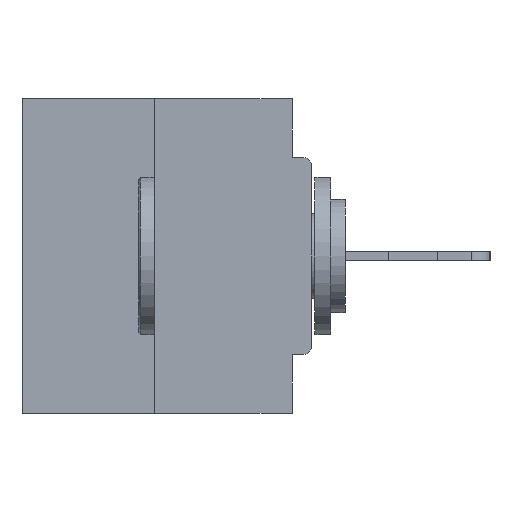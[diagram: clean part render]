
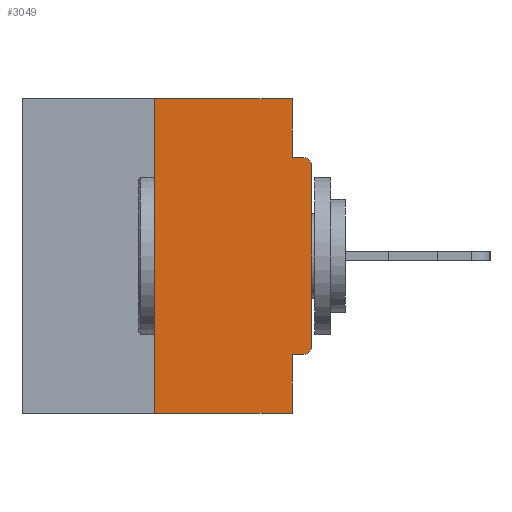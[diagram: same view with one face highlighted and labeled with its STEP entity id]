
A CAD part, left-side view. The second image highlights one B-rep face of the part: STEP entity #3049.
In plain terms, the highlighted planar face has unit normal (-1, 0, 0).
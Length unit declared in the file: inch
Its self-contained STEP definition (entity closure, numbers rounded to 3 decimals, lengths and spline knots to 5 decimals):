
#27 = DIRECTION ( 'NONE',  ( -1., 0., 0. ) ) ;
#231 = ORIENTED_EDGE ( 'NONE', *, *, #7795, .F. ) ;
#780 = VERTEX_POINT ( 'NONE', #21544 ) ;
#1097 = CARTESIAN_POINT ( 'NONE',  ( 0., 0., -0.1085 ) ) ;
#1395 = DIRECTION ( 'NONE',  ( 0., 1., 0. ) ) ;
#1961 = VERTEX_POINT ( 'NONE', #17027 ) ;
#2012 = ORIENTED_EDGE ( 'NONE', *, *, #29694, .F. ) ;
#2595 = AXIS2_PLACEMENT_3D ( 'NONE', #8878, #22515, #6292 ) ;
#3049 = ADVANCED_FACE ( 'NONE', ( #29610 ), #13852, .F. ) ;
#3472 = CIRCLE ( 'NONE', #5895, 0.015 ) ;
#3788 = CARTESIAN_POINT ( 'NONE',  ( 0., 0., -0.0935 ) ) ;
#3988 = VECTOR ( 'NONE', #19662, 39.37008 ) ;
#4588 = CARTESIAN_POINT ( 'NONE',  ( 0., 0.015, -0.1085 ) ) ;
#4682 = CARTESIAN_POINT ( 'NONE',  ( 0., 0.25, 0. ) ) ;
#4723 = DIRECTION ( 'NONE',  ( 0., 0., -1. ) ) ;
#5309 = VECTOR ( 'NONE', #21109, 39.37008 ) ;
#5895 = AXIS2_PLACEMENT_3D ( 'NONE', #4588, #27, #4723 ) ;
#6025 = LINE ( 'NONE', #24496, #24641 ) ;
#6292 = DIRECTION ( 'NONE',  ( 0., 0., -1. ) ) ;
#6522 = DIRECTION ( 'NONE',  ( 0., -1., 0. ) ) ;
#6960 = DIRECTION ( 'NONE',  ( 0., 0., 1. ) ) ;
#7469 = ORIENTED_EDGE ( 'NONE', *, *, #28873, .T. ) ;
#7495 = CARTESIAN_POINT ( 'NONE',  ( 0., 0.031, -0.5 ) ) ;
#7795 = EDGE_CURVE ( 'NONE', #17974, #28939, #20951, .T. ) ;
#8878 = CARTESIAN_POINT ( 'NONE',  ( 0., 0.015, -0.3915 ) ) ;
#8958 = VECTOR ( 'NONE', #6522, 39.37008 ) ;
#9535 = VERTEX_POINT ( 'NONE', #1097 ) ;
#9599 = CARTESIAN_POINT ( 'NONE',  ( 0., 0.46, 0. ) ) ;
#10550 = EDGE_CURVE ( 'NONE', #14853, #29250, #29198, .T. ) ;
#11734 = CARTESIAN_POINT ( 'NONE',  ( 0., 0.46, 0. ) ) ;
#12317 = ORIENTED_EDGE ( 'NONE', *, *, #26937, .T. ) ;
#13119 = DIRECTION ( 'NONE',  ( 0., 0., 1. ) ) ;
#13852 = PLANE ( 'NONE',  #20793 ) ;
#14151 = DIRECTION ( 'NONE',  ( 1., 0., 0. ) ) ;
#14847 = EDGE_CURVE ( 'NONE', #1961, #14853, #21865, .T. ) ;
#14853 = VERTEX_POINT ( 'NONE', #23837 ) ;
#15215 = LINE ( 'NONE', #26261, #18508 ) ;
#15325 = LINE ( 'NONE', #3788, #8958 ) ;
#15389 = EDGE_CURVE ( 'NONE', #17050, #28939, #6025, .T. ) ;
#15542 = LINE ( 'NONE', #15692, #16147 ) ;
#15692 = CARTESIAN_POINT ( 'NONE',  ( 0., 0., 0. ) ) ;
#15935 = CARTESIAN_POINT ( 'NONE',  ( 0., 0.25, -0.5 ) ) ;
#16147 = VECTOR ( 'NONE', #13119, 39.37008 ) ;
#16405 = VECTOR ( 'NONE', #16721, 39.37008 ) ;
#16721 = DIRECTION ( 'NONE',  ( 0., -1., 0. ) ) ;
#17027 = CARTESIAN_POINT ( 'NONE',  ( 0., 0.25, 0. ) ) ;
#17050 = VERTEX_POINT ( 'NONE', #15935 ) ;
#17974 = VERTEX_POINT ( 'NONE', #18708 ) ;
#17991 = DIRECTION ( 'NONE',  ( 0., -1., 0. ) ) ;
#18107 = CIRCLE ( 'NONE', #2595, 0.015 ) ;
#18137 = EDGE_CURVE ( 'NONE', #24770, #17974, #15215, .T. ) ;
#18480 = LINE ( 'NONE', #4682, #21465 ) ;
#18508 = VECTOR ( 'NONE', #1395, 39.37008 ) ;
#18692 = CARTESIAN_POINT ( 'NONE',  ( 0., 0.031, -0.5 ) ) ;
#18708 = CARTESIAN_POINT ( 'NONE',  ( 0., 0.031, -0.4065 ) ) ;
#18884 = EDGE_CURVE ( 'NONE', #17050, #1961, #18480, .T. ) ;
#19662 = DIRECTION ( 'NONE',  ( 0., 0., -1. ) ) ;
#20793 = AXIS2_PLACEMENT_3D ( 'NONE', #11734, #14151, #20970 ) ;
#20939 = VERTEX_POINT ( 'NONE', #27871 ) ;
#20951 = LINE ( 'NONE', #18692, #5309 ) ;
#20970 = DIRECTION ( 'NONE',  ( 0., 0., -1. ) ) ;
#21109 = DIRECTION ( 'NONE',  ( 0., 0., -1. ) ) ;
#21465 = VECTOR ( 'NONE', #6960, 39.37008 ) ;
#21544 = CARTESIAN_POINT ( 'NONE',  ( 0., 0., -0.3915 ) ) ;
#21865 = LINE ( 'NONE', #9599, #16405 ) ;
#22515 = DIRECTION ( 'NONE',  ( -1., 0., 0. ) ) ;
#23837 = CARTESIAN_POINT ( 'NONE',  ( 0., 0.031, 0. ) ) ;
#23899 = ORIENTED_EDGE ( 'NONE', *, *, #18884, .F. ) ;
#24052 = CARTESIAN_POINT ( 'NONE',  ( 0., 0.031, 0. ) ) ;
#24496 = CARTESIAN_POINT ( 'NONE',  ( 0., 0.46, -0.5 ) ) ;
#24641 = VECTOR ( 'NONE', #17991, 39.37008 ) ;
#24726 = CARTESIAN_POINT ( 'NONE',  ( 0., 0.031, -0.0935 ) ) ;
#24770 = VERTEX_POINT ( 'NONE', #27964 ) ;
#25485 = ORIENTED_EDGE ( 'NONE', *, *, #28832, .T. ) ;
#26261 = CARTESIAN_POINT ( 'NONE',  ( 0., 0., -0.4065 ) ) ;
#26679 = ORIENTED_EDGE ( 'NONE', *, *, #10550, .F. ) ;
#26937 = EDGE_CURVE ( 'NONE', #9535, #20939, #3472, .T. ) ;
#27421 = ORIENTED_EDGE ( 'NONE', *, *, #14847, .F. ) ;
#27871 = CARTESIAN_POINT ( 'NONE',  ( 0., 0.015, -0.0935 ) ) ;
#27964 = CARTESIAN_POINT ( 'NONE',  ( 0., 0.015, -0.4065 ) ) ;
#28832 = EDGE_CURVE ( 'NONE', #24770, #780, #18107, .T. ) ;
#28873 = EDGE_CURVE ( 'NONE', #780, #9535, #15542, .T. ) ;
#28939 = VERTEX_POINT ( 'NONE', #7495 ) ;
#28974 = ORIENTED_EDGE ( 'NONE', *, *, #18137, .F. ) ;
#29099 = EDGE_LOOP ( 'NONE', ( #27421, #23899, #29550, #231, #28974, #25485, #7469, #12317, #2012, #26679 ) ) ;
#29198 = LINE ( 'NONE', #24052, #3988 ) ;
#29250 = VERTEX_POINT ( 'NONE', #24726 ) ;
#29550 = ORIENTED_EDGE ( 'NONE', *, *, #15389, .T. ) ;
#29610 = FACE_OUTER_BOUND ( 'NONE', #29099, .T. ) ;
#29694 = EDGE_CURVE ( 'NONE', #29250, #20939, #15325, .T. ) ;
